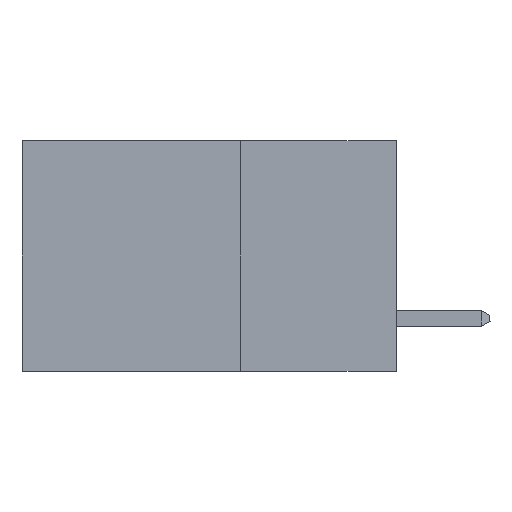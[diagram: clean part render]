
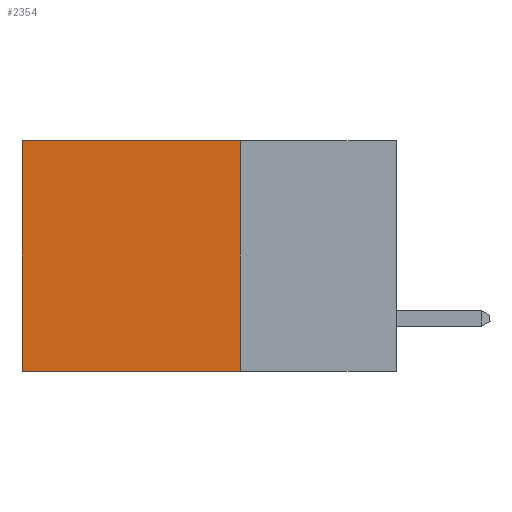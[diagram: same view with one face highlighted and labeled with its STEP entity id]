
A CAD part, left-side view. The second image highlights one B-rep face of the part: STEP entity #2354.
In plain terms, the highlighted planar face has unit normal (-1, 0, 0).
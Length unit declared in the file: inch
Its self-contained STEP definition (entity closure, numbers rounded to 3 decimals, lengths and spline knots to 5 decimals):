
#49 = CARTESIAN_POINT ( 'NONE',  ( 0.298, 0.25, -0.37 ) ) ;
#918 = LINE ( 'NONE', #1054, #10617 ) ;
#1054 = CARTESIAN_POINT ( 'NONE',  ( 0.298, 0.25, 0. ) ) ;
#1329 = AXIS2_PLACEMENT_3D ( 'NONE', #1476, #14071, #10677 ) ;
#1476 = CARTESIAN_POINT ( 'NONE',  ( 0.298, 0.25, 0. ) ) ;
#1667 = FACE_OUTER_BOUND ( 'NONE', #3742, .T. ) ;
#1778 = VERTEX_POINT ( 'NONE', #2971 ) ;
#1876 = DIRECTION ( 'NONE',  ( 0., 0., -1. ) ) ;
#2228 = CARTESIAN_POINT ( 'NONE',  ( 0.298, 0.25, 0. ) ) ;
#2354 = ADVANCED_FACE ( 'NONE', ( #1667 ), #7078, .F. ) ;
#2971 = CARTESIAN_POINT ( 'NONE',  ( 0.298, 0.6, 0. ) ) ;
#3742 = EDGE_LOOP ( 'NONE', ( #10064, #14266, #11029, #14160 ) ) ;
#4715 = VECTOR ( 'NONE', #11439, 39.37008 ) ;
#5610 = DIRECTION ( 'NONE',  ( 0., 0., -1. ) ) ;
#5708 = VERTEX_POINT ( 'NONE', #11605 ) ;
#5733 = LINE ( 'NONE', #14220, #11031 ) ;
#6207 = LINE ( 'NONE', #2228, #8837 ) ;
#6777 = DIRECTION ( 'NONE',  ( 0., 1., 0. ) ) ;
#6987 = LINE ( 'NONE', #49, #4715 ) ;
#7078 = PLANE ( 'NONE',  #1329 ) ;
#7717 = VERTEX_POINT ( 'NONE', #13431 ) ;
#7750 = EDGE_CURVE ( 'NONE', #5708, #1778, #6207, .T. ) ;
#8837 = VECTOR ( 'NONE', #6777, 39.37008 ) ;
#10064 = ORIENTED_EDGE ( 'NONE', *, *, #10510, .T. ) ;
#10510 = EDGE_CURVE ( 'NONE', #1778, #7717, #5733, .T. ) ;
#10617 = VECTOR ( 'NONE', #5610, 39.37008 ) ;
#10677 = DIRECTION ( 'NONE',  ( 0., 0., -1. ) ) ;
#11029 = ORIENTED_EDGE ( 'NONE', *, *, #11711, .F. ) ;
#11031 = VECTOR ( 'NONE', #1876, 39.37008 ) ;
#11439 = DIRECTION ( 'NONE',  ( 0., 1., 0. ) ) ;
#11605 = CARTESIAN_POINT ( 'NONE',  ( 0.298, 0.25, 0. ) ) ;
#11711 = EDGE_CURVE ( 'NONE', #5708, #12457, #918, .T. ) ;
#12457 = VERTEX_POINT ( 'NONE', #14481 ) ;
#13431 = CARTESIAN_POINT ( 'NONE',  ( 0.298, 0.6, -0.37 ) ) ;
#14013 = EDGE_CURVE ( 'NONE', #12457, #7717, #6987, .T. ) ;
#14071 = DIRECTION ( 'NONE',  ( 1., 0., 0. ) ) ;
#14160 = ORIENTED_EDGE ( 'NONE', *, *, #7750, .T. ) ;
#14220 = CARTESIAN_POINT ( 'NONE',  ( 0.298, 0.6, 0. ) ) ;
#14266 = ORIENTED_EDGE ( 'NONE', *, *, #14013, .F. ) ;
#14481 = CARTESIAN_POINT ( 'NONE',  ( 0.298, 0.25, -0.37 ) ) ;
